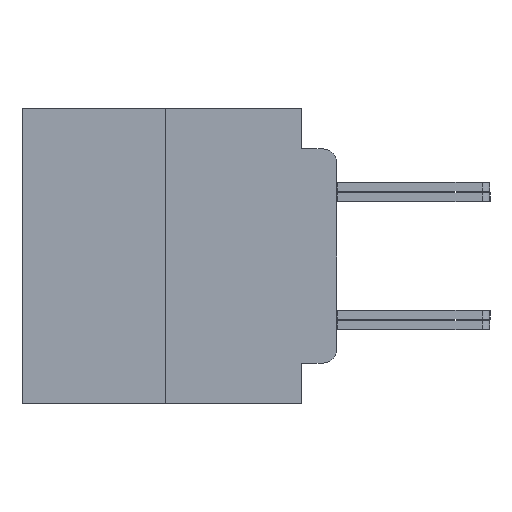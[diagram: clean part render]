
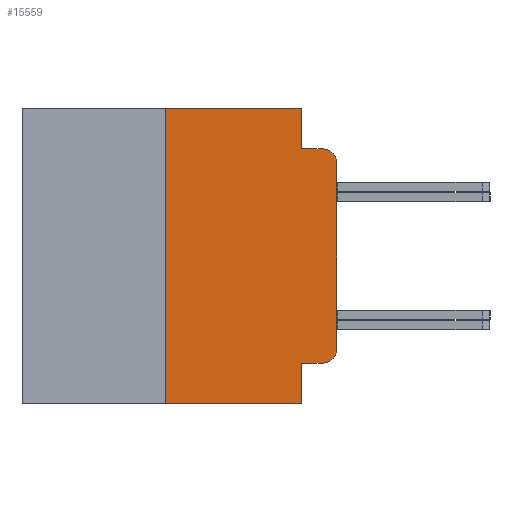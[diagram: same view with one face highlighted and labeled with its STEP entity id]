
A CAD part, left-side view. The second image highlights one B-rep face of the part: STEP entity #15559.
In plain terms, the highlighted planar face has unit normal (-1, 0, 0).
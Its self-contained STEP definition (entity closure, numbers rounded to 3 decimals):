
#1192 = CARTESIAN_POINT ( 'NONE',  ( -75.603, 1.295, 0. ) ) ;
#2527 = CARTESIAN_POINT ( 'NONE',  ( -75.603, 1.295, 3.975 ) ) ;
#3104 = ORIENTED_EDGE ( 'NONE', *, *, #24991, .F. ) ;
#3849 = VECTOR ( 'NONE', #25469, 1000. ) ;
#3902 = EDGE_CURVE ( 'NONE', #28405, #19522, #5560, .T. ) ;
#4289 = DIRECTION ( 'NONE',  ( -1., 0., 0. ) ) ;
#4395 = EDGE_LOOP ( 'NONE', ( #12854, #24513, #27669, #17873, #21155, #26104, #3104, #15772, #7803, #24040 ) ) ;
#4514 = EDGE_CURVE ( 'NONE', #19522, #20165, #5875, .T. ) ;
#4553 = EDGE_CURVE ( 'NONE', #6270, #20165, #17633, .T. ) ;
#5184 = CARTESIAN_POINT ( 'NONE',  ( -75.603, 6.35, 5.486 ) ) ;
#5233 = DIRECTION ( 'NONE',  ( 0., 0., -1. ) ) ;
#5537 = CARTESIAN_POINT ( 'NONE',  ( -75.603, 1.295, -3.975 ) ) ;
#5560 = LINE ( 'NONE', #6252, #26256 ) ;
#5712 = CARTESIAN_POINT ( 'NONE',  ( -75.603, 0.508, -3.975 ) ) ;
#5875 = CIRCLE ( 'NONE', #10065, 0.508 ) ;
#6080 = VERTEX_POINT ( 'NONE', #12863 ) ;
#6159 = EDGE_CURVE ( 'NONE', #6080, #20354, #20329, .T. ) ;
#6252 = CARTESIAN_POINT ( 'NONE',  ( -75.603, 0., 5.486 ) ) ;
#6270 = VERTEX_POINT ( 'NONE', #7009 ) ;
#6492 = DIRECTION ( 'NONE',  ( 0., 0., -1. ) ) ;
#6567 = VECTOR ( 'NONE', #14332, 1000. ) ;
#7009 = CARTESIAN_POINT ( 'NONE',  ( -75.603, 1.295, 3.975 ) ) ;
#7629 = DIRECTION ( 'NONE',  ( 1., 0., 0. ) ) ;
#7803 = ORIENTED_EDGE ( 'NONE', *, *, #26648, .T. ) ;
#9979 = CARTESIAN_POINT ( 'NONE',  ( -75.603, 6.35, -5.486 ) ) ;
#10065 = AXIS2_PLACEMENT_3D ( 'NONE', #17511, #4289, #6492 ) ;
#10677 = CARTESIAN_POINT ( 'NONE',  ( -75.603, 0., 3.467 ) ) ;
#11024 = VERTEX_POINT ( 'NONE', #9979 ) ;
#11058 = EDGE_CURVE ( 'NONE', #6080, #15603, #13144, .T. ) ;
#11083 = VECTOR ( 'NONE', #20206, 1000. ) ;
#11338 = CARTESIAN_POINT ( 'NONE',  ( -75.603, 1.295, 5.486 ) ) ;
#11486 = DIRECTION ( 'NONE',  ( 0., -1., 0. ) ) ;
#11700 = CARTESIAN_POINT ( 'NONE',  ( -75.603, 0.508, -3.467 ) ) ;
#11885 = DIRECTION ( 'NONE',  ( 0., 0., -1. ) ) ;
#12127 = VERTEX_POINT ( 'NONE', #11338 ) ;
#12854 = ORIENTED_EDGE ( 'NONE', *, *, #11058, .T. ) ;
#12863 = CARTESIAN_POINT ( 'NONE',  ( -75.603, 1.295, -3.975 ) ) ;
#13144 = LINE ( 'NONE', #5537, #6567 ) ;
#13973 = VECTOR ( 'NONE', #16628, 1000. ) ;
#14332 = DIRECTION ( 'NONE',  ( 0., -1., 0. ) ) ;
#14450 = VECTOR ( 'NONE', #15381, 1000. ) ;
#15381 = DIRECTION ( 'NONE',  ( 0., 0., -1. ) ) ;
#15559 = ADVANCED_FACE ( 'NONE', ( #20230 ), #16255, .F. ) ;
#15603 = VERTEX_POINT ( 'NONE', #5712 ) ;
#15772 = ORIENTED_EDGE ( 'NONE', *, *, #24779, .F. ) ;
#16255 = PLANE ( 'NONE',  #23115 ) ;
#16541 = VECTOR ( 'NONE', #11486, 1000. ) ;
#16628 = DIRECTION ( 'NONE',  ( 0., 0., -1. ) ) ;
#17511 = CARTESIAN_POINT ( 'NONE',  ( -75.603, 0.508, 3.467 ) ) ;
#17633 = LINE ( 'NONE', #2527, #11083 ) ;
#17873 = ORIENTED_EDGE ( 'NONE', *, *, #4514, .T. ) ;
#18033 = AXIS2_PLACEMENT_3D ( 'NONE', #11700, #25301, #11885 ) ;
#18342 = CARTESIAN_POINT ( 'NONE',  ( -75.603, 11.684, 5.486 ) ) ;
#18473 = CARTESIAN_POINT ( 'NONE',  ( -75.603, 11.684, 5.486 ) ) ;
#18535 = CARTESIAN_POINT ( 'NONE',  ( -75.603, 1.295, -5.486 ) ) ;
#18962 = LINE ( 'NONE', #20180, #16541 ) ;
#19070 = LINE ( 'NONE', #20387, #25942 ) ;
#19522 = VERTEX_POINT ( 'NONE', #10677 ) ;
#19913 = CARTESIAN_POINT ( 'NONE',  ( -75.603, 1.295, 0. ) ) ;
#20165 = VERTEX_POINT ( 'NONE', #22134 ) ;
#20180 = CARTESIAN_POINT ( 'NONE',  ( -75.603, 11.684, -5.486 ) ) ;
#20206 = DIRECTION ( 'NONE',  ( 0., -1., 0. ) ) ;
#20230 = FACE_OUTER_BOUND ( 'NONE', #4395, .T. ) ;
#20329 = LINE ( 'NONE', #19913, #14450 ) ;
#20354 = VERTEX_POINT ( 'NONE', #18535 ) ;
#20387 = CARTESIAN_POINT ( 'NONE',  ( -75.603, 6.35, -5.486 ) ) ;
#21155 = ORIENTED_EDGE ( 'NONE', *, *, #4553, .F. ) ;
#22134 = CARTESIAN_POINT ( 'NONE',  ( -75.603, 0.508, 3.975 ) ) ;
#23115 = AXIS2_PLACEMENT_3D ( 'NONE', #18473, #7629, #5233 ) ;
#23306 = EDGE_CURVE ( 'NONE', #12127, #6270, #24690, .T. ) ;
#23916 = CARTESIAN_POINT ( 'NONE',  ( -75.603, 0., -3.467 ) ) ;
#24040 = ORIENTED_EDGE ( 'NONE', *, *, #6159, .F. ) ;
#24513 = ORIENTED_EDGE ( 'NONE', *, *, #27461, .T. ) ;
#24690 = LINE ( 'NONE', #1192, #13973 ) ;
#24779 = EDGE_CURVE ( 'NONE', #11024, #28065, #19070, .T. ) ;
#24991 = EDGE_CURVE ( 'NONE', #28065, #12127, #27672, .T. ) ;
#25301 = DIRECTION ( 'NONE',  ( -1., 0., 0. ) ) ;
#25469 = DIRECTION ( 'NONE',  ( 0., -1., 0. ) ) ;
#25942 = VECTOR ( 'NONE', #26716, 1000. ) ;
#26104 = ORIENTED_EDGE ( 'NONE', *, *, #23306, .F. ) ;
#26126 = DIRECTION ( 'NONE',  ( 0., 0., 1. ) ) ;
#26256 = VECTOR ( 'NONE', #26126, 1000. ) ;
#26648 = EDGE_CURVE ( 'NONE', #11024, #20354, #18962, .T. ) ;
#26716 = DIRECTION ( 'NONE',  ( 0., 0., 1. ) ) ;
#27461 = EDGE_CURVE ( 'NONE', #15603, #28405, #27880, .T. ) ;
#27669 = ORIENTED_EDGE ( 'NONE', *, *, #3902, .T. ) ;
#27672 = LINE ( 'NONE', #18342, #3849 ) ;
#27880 = CIRCLE ( 'NONE', #18033, 0.508 ) ;
#28065 = VERTEX_POINT ( 'NONE', #5184 ) ;
#28405 = VERTEX_POINT ( 'NONE', #23916 ) ;
